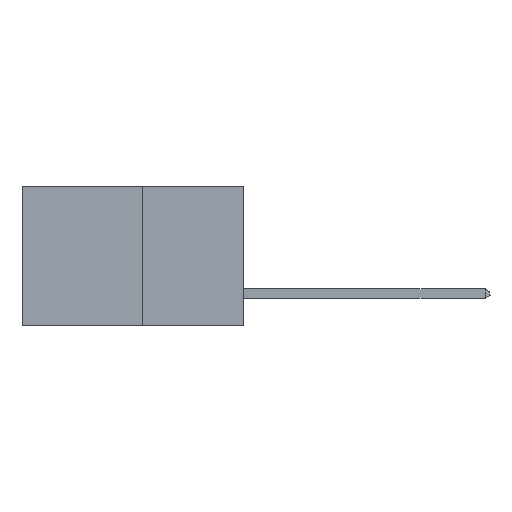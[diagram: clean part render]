
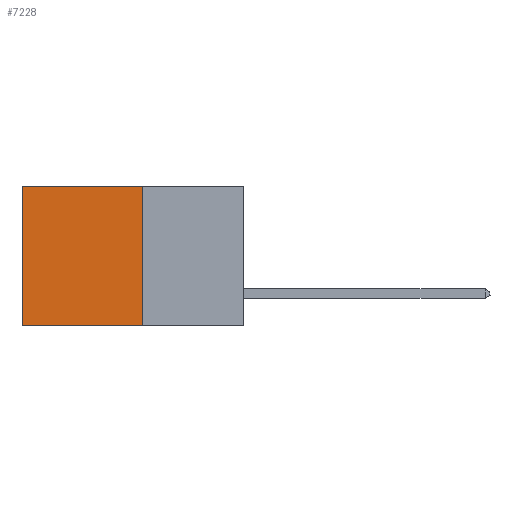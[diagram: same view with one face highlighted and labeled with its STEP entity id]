
A CAD part, left-side view. The second image highlights one B-rep face of the part: STEP entity #7228.
In plain terms, the highlighted planar face has unit normal (-1, 0, 0).
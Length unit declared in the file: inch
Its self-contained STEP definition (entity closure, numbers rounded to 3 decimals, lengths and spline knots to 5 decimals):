
#319 = AXIS2_PLACEMENT_3D ( 'NONE', #14991, #14965, #14855 ) ;
#522 = CARTESIAN_POINT ( 'NONE',  ( 0.277, 0.59, -0.37 ) ) ;
#1795 = DIRECTION ( 'NONE',  ( 0., 1., 0. ) ) ;
#2075 = ORIENTED_EDGE ( 'NONE', *, *, #8830, .T. ) ;
#2312 = VERTEX_POINT ( 'NONE', #16456 ) ;
#2610 = DIRECTION ( 'NONE',  ( 0., 0., -1. ) ) ;
#3713 = LINE ( 'NONE', #522, #14015 ) ;
#3968 = EDGE_LOOP ( 'NONE', ( #19792, #5966, #5438, #2075 ) ) ;
#5235 = VECTOR ( 'NONE', #23450, 39.37008 ) ;
#5438 = ORIENTED_EDGE ( 'NONE', *, *, #11838, .F. ) ;
#5555 = DIRECTION ( 'NONE',  ( 0., 1., 0. ) ) ;
#5966 = ORIENTED_EDGE ( 'NONE', *, *, #16647, .F. ) ;
#7228 = ADVANCED_FACE ( 'NONE', ( #22092 ), #16318, .F. ) ;
#8830 = EDGE_CURVE ( 'NONE', #2312, #15559, #10904, .T. ) ;
#9341 = CARTESIAN_POINT ( 'NONE',  ( 0.277, 0.27, -0.37 ) ) ;
#10071 = LINE ( 'NONE', #9341, #5235 ) ;
#10252 = VECTOR ( 'NONE', #1795, 39.37008 ) ;
#10416 = EDGE_CURVE ( 'NONE', #15559, #11897, #3713, .T. ) ;
#10641 = CARTESIAN_POINT ( 'NONE',  ( 0.277, 0.59, 0. ) ) ;
#10904 = LINE ( 'NONE', #26028, #10252 ) ;
#11838 = EDGE_CURVE ( 'NONE', #2312, #18577, #10071, .T. ) ;
#11897 = VERTEX_POINT ( 'NONE', #21638 ) ;
#12933 = LINE ( 'NONE', #17806, #18356 ) ;
#14015 = VECTOR ( 'NONE', #2610, 39.37008 ) ;
#14855 = DIRECTION ( 'NONE',  ( 0., 0., -1. ) ) ;
#14965 = DIRECTION ( 'NONE',  ( 1., 0., 0. ) ) ;
#14991 = CARTESIAN_POINT ( 'NONE',  ( 0.277, 0.27, -0.37 ) ) ;
#15510 = CARTESIAN_POINT ( 'NONE',  ( 0.277, 0.27, -0.37 ) ) ;
#15559 = VERTEX_POINT ( 'NONE', #10641 ) ;
#16318 = PLANE ( 'NONE',  #319 ) ;
#16456 = CARTESIAN_POINT ( 'NONE',  ( 0.277, 0.27, 0. ) ) ;
#16647 = EDGE_CURVE ( 'NONE', #18577, #11897, #12933, .T. ) ;
#17806 = CARTESIAN_POINT ( 'NONE',  ( 0.277, 0.27, -0.37 ) ) ;
#18356 = VECTOR ( 'NONE', #5555, 39.37008 ) ;
#18577 = VERTEX_POINT ( 'NONE', #15510 ) ;
#19792 = ORIENTED_EDGE ( 'NONE', *, *, #10416, .T. ) ;
#21638 = CARTESIAN_POINT ( 'NONE',  ( 0.277, 0.59, -0.37 ) ) ;
#22092 = FACE_OUTER_BOUND ( 'NONE', #3968, .T. ) ;
#23450 = DIRECTION ( 'NONE',  ( 0., 0., -1. ) ) ;
#26028 = CARTESIAN_POINT ( 'NONE',  ( 0.277, 0.27, 0. ) ) ;
